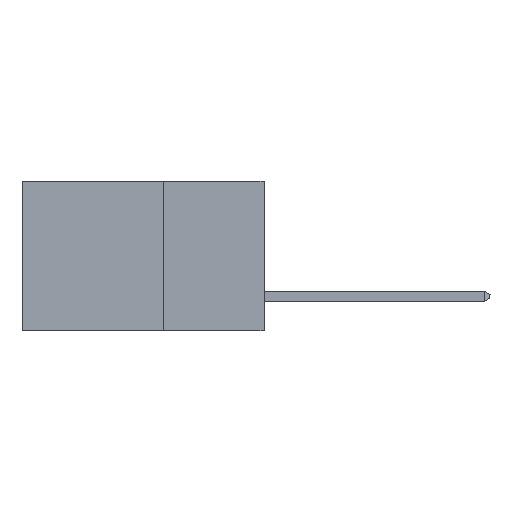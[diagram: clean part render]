
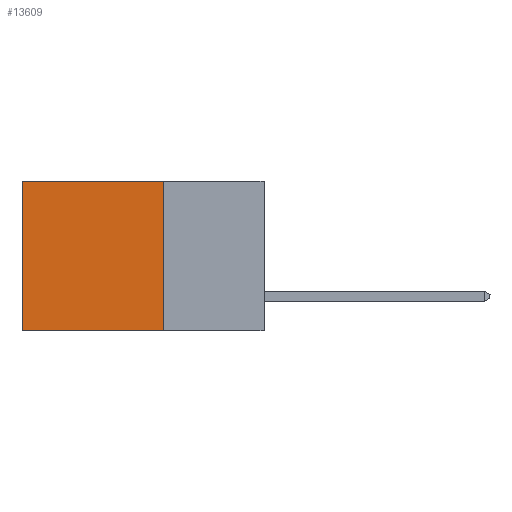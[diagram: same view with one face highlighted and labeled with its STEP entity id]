
A CAD part, left-side view. The second image highlights one B-rep face of the part: STEP entity #13609.
In plain terms, the highlighted planar face has unit normal (-1, 0, 0).
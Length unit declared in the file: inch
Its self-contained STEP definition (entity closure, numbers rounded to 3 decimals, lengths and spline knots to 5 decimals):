
#214 = CARTESIAN_POINT ( 'NONE',  ( 0.2615, 0.25, -0.37 ) ) ;
#1132 = EDGE_CURVE ( 'NONE', #1967, #3484, #6596, .T. ) ;
#1967 = VERTEX_POINT ( 'NONE', #15165 ) ;
#2854 = DIRECTION ( 'NONE',  ( 0., 0., -1. ) ) ;
#3484 = VERTEX_POINT ( 'NONE', #6282 ) ;
#4210 = EDGE_CURVE ( 'NONE', #23020, #3484, #17034, .T. ) ;
#4330 = CARTESIAN_POINT ( 'NONE',  ( 0.2615, 0.25, -0.37 ) ) ;
#4964 = LINE ( 'NONE', #16286, #22913 ) ;
#5318 = VECTOR ( 'NONE', #23545, 39.37008 ) ;
#6282 = CARTESIAN_POINT ( 'NONE',  ( 0.2615, 0.6, -0.37 ) ) ;
#6596 = LINE ( 'NONE', #6956, #5318 ) ;
#6956 = CARTESIAN_POINT ( 'NONE',  ( 0.2615, 0.6, -0.37 ) ) ;
#6978 = EDGE_CURVE ( 'NONE', #20279, #23020, #16920, .T. ) ;
#7481 = ORIENTED_EDGE ( 'NONE', *, *, #6978, .F. ) ;
#7703 = DIRECTION ( 'NONE',  ( 0., 1., 0. ) ) ;
#8027 = VECTOR ( 'NONE', #7703, 39.37008 ) ;
#8404 = AXIS2_PLACEMENT_3D ( 'NONE', #4330, #19572, #2854 ) ;
#9307 = CARTESIAN_POINT ( 'NONE',  ( 0.2615, 0.25, -0.37 ) ) ;
#9921 = EDGE_LOOP ( 'NONE', ( #23314, #23067, #7481, #15569 ) ) ;
#10104 = PLANE ( 'NONE',  #8404 ) ;
#10867 = VECTOR ( 'NONE', #20479, 39.37008 ) ;
#11287 = CARTESIAN_POINT ( 'NONE',  ( 0.2615, 0.25, 0. ) ) ;
#13609 = ADVANCED_FACE ( 'NONE', ( #14048 ), #10104, .F. ) ;
#14048 = FACE_OUTER_BOUND ( 'NONE', #9921, .T. ) ;
#14440 = DIRECTION ( 'NONE',  ( 0., 1., 0. ) ) ;
#15165 = CARTESIAN_POINT ( 'NONE',  ( 0.2615, 0.6, 0. ) ) ;
#15569 = ORIENTED_EDGE ( 'NONE', *, *, #22368, .T. ) ;
#16286 = CARTESIAN_POINT ( 'NONE',  ( 0.2615, 0.25, 0. ) ) ;
#16920 = LINE ( 'NONE', #9307, #10867 ) ;
#17034 = LINE ( 'NONE', #214, #8027 ) ;
#19572 = DIRECTION ( 'NONE',  ( 1., 0., 0. ) ) ;
#20279 = VERTEX_POINT ( 'NONE', #11287 ) ;
#20479 = DIRECTION ( 'NONE',  ( 0., 0., -1. ) ) ;
#21955 = CARTESIAN_POINT ( 'NONE',  ( 0.2615, 0.25, -0.37 ) ) ;
#22368 = EDGE_CURVE ( 'NONE', #20279, #1967, #4964, .T. ) ;
#22913 = VECTOR ( 'NONE', #14440, 39.37008 ) ;
#23020 = VERTEX_POINT ( 'NONE', #21955 ) ;
#23067 = ORIENTED_EDGE ( 'NONE', *, *, #4210, .F. ) ;
#23314 = ORIENTED_EDGE ( 'NONE', *, *, #1132, .T. ) ;
#23545 = DIRECTION ( 'NONE',  ( 0., 0., -1. ) ) ;
